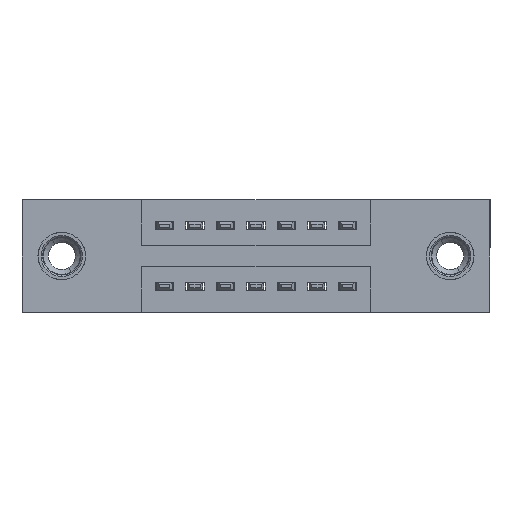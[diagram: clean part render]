
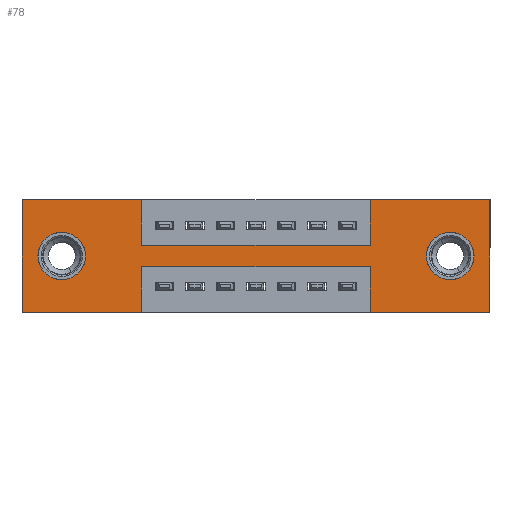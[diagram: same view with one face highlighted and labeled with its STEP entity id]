
A CAD part, front view. The second image highlights one B-rep face of the part: STEP entity #78.
In plain terms, the highlighted planar face has unit normal (0, -1, 0).
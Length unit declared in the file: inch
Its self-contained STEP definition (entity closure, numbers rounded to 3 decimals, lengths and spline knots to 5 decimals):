
#78 = ADVANCED_FACE ( 'NONE', ( #445, #5341, #3104 ), #1982, .T. ) ;
#196 = LINE ( 'NONE', #7480, #7545 ) ;
#335 = LINE ( 'NONE', #11567, #10116 ) ;
#378 = VECTOR ( 'NONE', #7701, 39.37008 ) ;
#422 = CARTESIAN_POINT ( 'NONE',  ( 1.1425, 0., 0. ) ) ;
#445 = FACE_BOUND ( 'NONE', #10059, .T. ) ;
#505 = DIRECTION ( 'NONE',  ( 0., 1., 0. ) ) ;
#525 = DIRECTION ( 'NONE',  ( 0., 0., 1. ) ) ;
#558 = LINE ( 'NONE', #422, #10323 ) ;
#601 = AXIS2_PLACEMENT_3D ( 'NONE', #3355, #9860, #4341 ) ;
#699 = EDGE_CURVE ( 'NONE', #5249, #11669, #11763, .T. ) ;
#785 = VERTEX_POINT ( 'NONE', #8261 ) ;
#970 = CARTESIAN_POINT ( 'NONE',  ( 1.1425, 0., 0. ) ) ;
#1031 = AXIS2_PLACEMENT_3D ( 'NONE', #2284, #11008, #7257 ) ;
#1093 = EDGE_CURVE ( 'NONE', #11260, #785, #5902, .T. ) ;
#1225 = VERTEX_POINT ( 'NONE', #9008 ) ;
#1234 = EDGE_CURVE ( 'NONE', #4773, #5554, #1854, .T. ) ;
#1311 = DIRECTION ( 'NONE',  ( -1., 0., 0. ) ) ;
#1642 = CARTESIAN_POINT ( 'NONE',  ( 0., 0., 0. ) ) ;
#1653 = ORIENTED_EDGE ( 'NONE', *, *, #1855, .F. ) ;
#1678 = VECTOR ( 'NONE', #2632, 39.37008 ) ;
#1798 = DIRECTION ( 'NONE',  ( 1., 0., 0. ) ) ;
#1854 = CIRCLE ( 'NONE', #8611, 0.078 ) ;
#1855 = EDGE_CURVE ( 'NONE', #11518, #3736, #558, .T. ) ;
#1914 = ORIENTED_EDGE ( 'NONE', *, *, #3005, .F. ) ;
#1982 = PLANE ( 'NONE',  #1031 ) ;
#2040 = ORIENTED_EDGE ( 'NONE', *, *, #5094, .F. ) ;
#2208 = ORIENTED_EDGE ( 'NONE', *, *, #2587, .F. ) ;
#2209 = VERTEX_POINT ( 'NONE', #9994 ) ;
#2284 = CARTESIAN_POINT ( 'NONE',  ( 0., 0., -0.37 ) ) ;
#2416 = CARTESIAN_POINT ( 'NONE',  ( 0.3925, 0., -0.37 ) ) ;
#2494 = EDGE_CURVE ( 'NONE', #2902, #1225, #8582, .T. ) ;
#2587 = EDGE_CURVE ( 'NONE', #9996, #9608, #7987, .T. ) ;
#2632 = DIRECTION ( 'NONE',  ( 1., 0., 0. ) ) ;
#2856 = ORIENTED_EDGE ( 'NONE', *, *, #3013, .T. ) ;
#2902 = VERTEX_POINT ( 'NONE', #4964 ) ;
#2944 = CARTESIAN_POINT ( 'NONE',  ( 0.13, 0., -0.263 ) ) ;
#3005 = EDGE_CURVE ( 'NONE', #2209, #6726, #9155, .T. ) ;
#3013 = EDGE_CURVE ( 'NONE', #11669, #5249, #8854, .T. ) ;
#3051 = VECTOR ( 'NONE', #10506, 39.37008 ) ;
#3080 = VECTOR ( 'NONE', #10366, 39.37008 ) ;
#3104 = FACE_OUTER_BOUND ( 'NONE', #4071, .T. ) ;
#3116 = ORIENTED_EDGE ( 'NONE', *, *, #8292, .F. ) ;
#3126 = DIRECTION ( 'NONE',  ( 0., 0., -1. ) ) ;
#3239 = VECTOR ( 'NONE', #1798, 39.37008 ) ;
#3310 = EDGE_CURVE ( 'NONE', #9608, #11518, #4990, .T. ) ;
#3355 = CARTESIAN_POINT ( 'NONE',  ( 0.13, 0., -0.185 ) ) ;
#3409 = CARTESIAN_POINT ( 'NONE',  ( 0.3925, 0., 0. ) ) ;
#3710 = ORIENTED_EDGE ( 'NONE', *, *, #1093, .F. ) ;
#3736 = VERTEX_POINT ( 'NONE', #970 ) ;
#3788 = ORIENTED_EDGE ( 'NONE', *, *, #1234, .T. ) ;
#4012 = EDGE_CURVE ( 'NONE', #785, #8659, #196, .T. ) ;
#4071 = EDGE_LOOP ( 'NONE', ( #7774, #8961, #5924, #7370, #3710, #3116, #1653, #8381, #2208, #5436, #1914, #2040 ) ) ;
#4124 = ORIENTED_EDGE ( 'NONE', *, *, #699, .T. ) ;
#4258 = VECTOR ( 'NONE', #11019, 39.37008 ) ;
#4341 = DIRECTION ( 'NONE',  ( 0., 0., 1. ) ) ;
#4534 = VECTOR ( 'NONE', #6194, 39.37008 ) ;
#4541 = EDGE_CURVE ( 'NONE', #8659, #11758, #9424, .T. ) ;
#4556 = CARTESIAN_POINT ( 'NONE',  ( 1.1425, 0., -0.15 ) ) ;
#4683 = CARTESIAN_POINT ( 'NONE',  ( 0.13, 0., -0.107 ) ) ;
#4773 = VERTEX_POINT ( 'NONE', #4683 ) ;
#4782 = AXIS2_PLACEMENT_3D ( 'NONE', #12127, #505, #5019 ) ;
#4874 = LINE ( 'NONE', #11170, #11882 ) ;
#4884 = CARTESIAN_POINT ( 'NONE',  ( 0., 0., 0. ) ) ;
#4964 = CARTESIAN_POINT ( 'NONE',  ( 0.3925, 0., -0.22 ) ) ;
#4990 = LINE ( 'NONE', #10531, #3051 ) ;
#5019 = DIRECTION ( 'NONE',  ( 0., 0., -1. ) ) ;
#5094 = EDGE_CURVE ( 'NONE', #1225, #2209, #335, .T. ) ;
#5249 = VERTEX_POINT ( 'NONE', #8156 ) ;
#5252 = CARTESIAN_POINT ( 'NONE',  ( 1.1425, 0., -0.37 ) ) ;
#5341 = FACE_BOUND ( 'NONE', #6706, .T. ) ;
#5436 = ORIENTED_EDGE ( 'NONE', *, *, #9376, .F. ) ;
#5554 = VERTEX_POINT ( 'NONE', #2944 ) ;
#5708 = EDGE_CURVE ( 'NONE', #5554, #4773, #6242, .T. ) ;
#5842 = CARTESIAN_POINT ( 'NONE',  ( 0.3925, 0., -0.15 ) ) ;
#5888 = LINE ( 'NONE', #10175, #3239 ) ;
#5902 = LINE ( 'NONE', #10502, #3080 ) ;
#5924 = ORIENTED_EDGE ( 'NONE', *, *, #4541, .F. ) ;
#6194 = DIRECTION ( 'NONE',  ( 0., 0., 1. ) ) ;
#6242 = CIRCLE ( 'NONE', #601, 0.078 ) ;
#6422 = CARTESIAN_POINT ( 'NONE',  ( 0.3925, 0., 0. ) ) ;
#6443 = VECTOR ( 'NONE', #3126, 39.37008 ) ;
#6599 = DIRECTION ( 'NONE',  ( -1., 0., 0. ) ) ;
#6706 = EDGE_LOOP ( 'NONE', ( #3788, #8601 ) ) ;
#6726 = VERTEX_POINT ( 'NONE', #4884 ) ;
#7257 = DIRECTION ( 'NONE',  ( 0., 0., -1. ) ) ;
#7370 = ORIENTED_EDGE ( 'NONE', *, *, #4012, .F. ) ;
#7463 = CARTESIAN_POINT ( 'NONE',  ( 1.405, 0., -0.263 ) ) ;
#7480 = CARTESIAN_POINT ( 'NONE',  ( 0., 0., -0.37 ) ) ;
#7545 = VECTOR ( 'NONE', #8164, 39.37008 ) ;
#7701 = DIRECTION ( 'NONE',  ( 0., 0., -1. ) ) ;
#7774 = ORIENTED_EDGE ( 'NONE', *, *, #2494, .F. ) ;
#7987 = LINE ( 'NONE', #3409, #378 ) ;
#8156 = CARTESIAN_POINT ( 'NONE',  ( 1.405, 0., -0.107 ) ) ;
#8164 = DIRECTION ( 'NONE',  ( -1., 0., 0. ) ) ;
#8261 = CARTESIAN_POINT ( 'NONE',  ( 1.535, 0., -0.37 ) ) ;
#8292 = EDGE_CURVE ( 'NONE', #3736, #11260, #5888, .T. ) ;
#8381 = ORIENTED_EDGE ( 'NONE', *, *, #3310, .F. ) ;
#8582 = LINE ( 'NONE', #2416, #6443 ) ;
#8601 = ORIENTED_EDGE ( 'NONE', *, *, #5708, .T. ) ;
#8608 = DIRECTION ( 'NONE',  ( 0., 0., 1. ) ) ;
#8611 = AXIS2_PLACEMENT_3D ( 'NONE', #8684, #8635, #8608 ) ;
#8635 = DIRECTION ( 'NONE',  ( 0., 1., 0. ) ) ;
#8659 = VERTEX_POINT ( 'NONE', #9868 ) ;
#8684 = CARTESIAN_POINT ( 'NONE',  ( 0.13, 0., -0.185 ) ) ;
#8723 = CARTESIAN_POINT ( 'NONE',  ( 1.535, 0., 0. ) ) ;
#8854 = CIRCLE ( 'NONE', #4782, 0.078 ) ;
#8961 = ORIENTED_EDGE ( 'NONE', *, *, #10141, .F. ) ;
#9008 = CARTESIAN_POINT ( 'NONE',  ( 0.3925, 0., -0.37 ) ) ;
#9155 = LINE ( 'NONE', #10688, #4258 ) ;
#9175 = LINE ( 'NONE', #1642, #1678 ) ;
#9376 = EDGE_CURVE ( 'NONE', #6726, #9996, #9175, .T. ) ;
#9424 = LINE ( 'NONE', #5252, #4534 ) ;
#9608 = VERTEX_POINT ( 'NONE', #5842 ) ;
#9860 = DIRECTION ( 'NONE',  ( 0., 1., 0. ) ) ;
#9868 = CARTESIAN_POINT ( 'NONE',  ( 1.1425, 0., -0.37 ) ) ;
#9994 = CARTESIAN_POINT ( 'NONE',  ( 0., 0., -0.37 ) ) ;
#9996 = VERTEX_POINT ( 'NONE', #6422 ) ;
#10059 = EDGE_LOOP ( 'NONE', ( #4124, #2856 ) ) ;
#10116 = VECTOR ( 'NONE', #1311, 39.37008 ) ;
#10141 = EDGE_CURVE ( 'NONE', #11758, #2902, #4874, .T. ) ;
#10175 = CARTESIAN_POINT ( 'NONE',  ( 0., 0., 0. ) ) ;
#10323 = VECTOR ( 'NONE', #525, 39.37008 ) ;
#10366 = DIRECTION ( 'NONE',  ( 0., 0., -1. ) ) ;
#10502 = CARTESIAN_POINT ( 'NONE',  ( 1.535, 0., 0. ) ) ;
#10506 = DIRECTION ( 'NONE',  ( 1., 0., 0. ) ) ;
#10531 = CARTESIAN_POINT ( 'NONE',  ( 0.3925, 0., -0.15 ) ) ;
#10676 = DIRECTION ( 'NONE',  ( 0., 0., -1. ) ) ;
#10688 = CARTESIAN_POINT ( 'NONE',  ( 0., 0., 0. ) ) ;
#10695 = DIRECTION ( 'NONE',  ( 0., 1., 0. ) ) ;
#10879 = CARTESIAN_POINT ( 'NONE',  ( 1.405, 0., -0.185 ) ) ;
#10885 = AXIS2_PLACEMENT_3D ( 'NONE', #10879, #10695, #10676 ) ;
#11008 = DIRECTION ( 'NONE',  ( 0., -1., 0. ) ) ;
#11019 = DIRECTION ( 'NONE',  ( 0., 0., 1. ) ) ;
#11170 = CARTESIAN_POINT ( 'NONE',  ( 0.3925, 0., -0.22 ) ) ;
#11260 = VERTEX_POINT ( 'NONE', #8723 ) ;
#11279 = CARTESIAN_POINT ( 'NONE',  ( 1.1425, 0., -0.22 ) ) ;
#11518 = VERTEX_POINT ( 'NONE', #4556 ) ;
#11567 = CARTESIAN_POINT ( 'NONE',  ( 0., 0., -0.37 ) ) ;
#11669 = VERTEX_POINT ( 'NONE', #7463 ) ;
#11758 = VERTEX_POINT ( 'NONE', #11279 ) ;
#11763 = CIRCLE ( 'NONE', #10885, 0.078 ) ;
#11882 = VECTOR ( 'NONE', #6599, 39.37008 ) ;
#12127 = CARTESIAN_POINT ( 'NONE',  ( 1.405, 0., -0.185 ) ) ;
